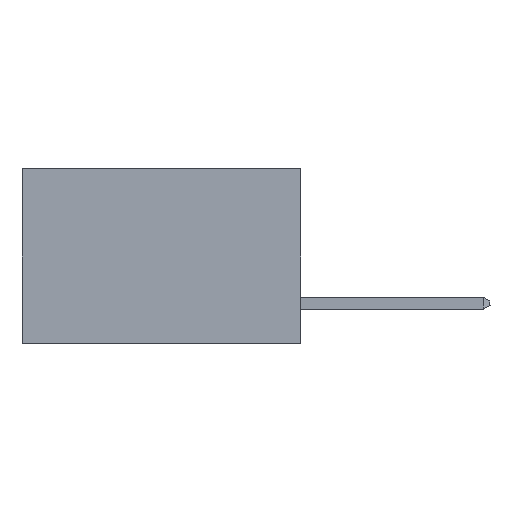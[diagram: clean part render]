
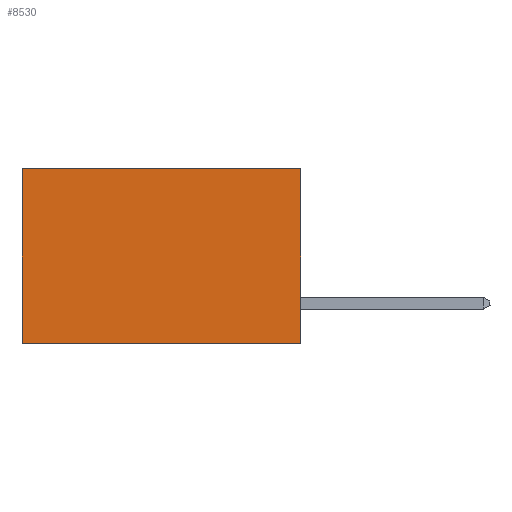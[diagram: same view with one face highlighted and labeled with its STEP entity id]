
A CAD part, left-side view. The second image highlights one B-rep face of the part: STEP entity #8530.
In plain terms, the highlighted planar face has unit normal (-1, 0, 0).
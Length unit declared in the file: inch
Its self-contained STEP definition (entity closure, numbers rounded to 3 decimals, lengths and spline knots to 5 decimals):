
#39 = ORIENTED_EDGE ( 'NONE', *, *, #13125, .T. ) ;
#360 = CARTESIAN_POINT ( 'NONE',  ( 0.277, 0.59, -0.37 ) ) ;
#2025 = CARTESIAN_POINT ( 'NONE',  ( 0.277, 0., -0.37 ) ) ;
#2088 = VECTOR ( 'NONE', #2269, 39.37008 ) ;
#2198 = CARTESIAN_POINT ( 'NONE',  ( 0.277, 0.59, 0. ) ) ;
#2269 = DIRECTION ( 'NONE',  ( 0., 0., -1. ) ) ;
#2933 = EDGE_CURVE ( 'NONE', #12472, #13410, #11295, .T. ) ;
#3009 = ORIENTED_EDGE ( 'NONE', *, *, #2933, .F. ) ;
#4418 = EDGE_CURVE ( 'NONE', #12472, #10656, #12048, .T. ) ;
#4995 = DIRECTION ( 'NONE',  ( 0., 0., -1. ) ) ;
#5043 = DIRECTION ( 'NONE',  ( 1., 0., 0. ) ) ;
#5099 = PLANE ( 'NONE',  #13318 ) ;
#5214 = CARTESIAN_POINT ( 'NONE',  ( 0.277, 0., -0.37 ) ) ;
#6611 = CARTESIAN_POINT ( 'NONE',  ( 0.277, 0., -0.37 ) ) ;
#7109 = CARTESIAN_POINT ( 'NONE',  ( 0.277, 0., -0.37 ) ) ;
#8530 = ADVANCED_FACE ( 'NONE', ( #11954 ), #5099, .F. ) ;
#9438 = CARTESIAN_POINT ( 'NONE',  ( 0.277, 0., 0. ) ) ;
#10656 = VERTEX_POINT ( 'NONE', #2198 ) ;
#11295 = LINE ( 'NONE', #2025, #11849 ) ;
#11760 = VECTOR ( 'NONE', #13800, 39.37008 ) ;
#11849 = VECTOR ( 'NONE', #16401, 39.37008 ) ;
#11954 = FACE_OUTER_BOUND ( 'NONE', #15161, .T. ) ;
#12048 = LINE ( 'NONE', #17544, #16717 ) ;
#12417 = ORIENTED_EDGE ( 'NONE', *, *, #13920, .F. ) ;
#12472 = VERTEX_POINT ( 'NONE', #9438 ) ;
#13125 = EDGE_CURVE ( 'NONE', #10656, #14734, #16491, .T. ) ;
#13318 = AXIS2_PLACEMENT_3D ( 'NONE', #5214, #5043, #4995 ) ;
#13410 = VERTEX_POINT ( 'NONE', #7109 ) ;
#13800 = DIRECTION ( 'NONE',  ( 0., 1., 0. ) ) ;
#13920 = EDGE_CURVE ( 'NONE', #13410, #14734, #21199, .T. ) ;
#14734 = VERTEX_POINT ( 'NONE', #22971 ) ;
#15161 = EDGE_LOOP ( 'NONE', ( #39, #12417, #3009, #23215 ) ) ;
#16401 = DIRECTION ( 'NONE',  ( 0., 0., -1. ) ) ;
#16491 = LINE ( 'NONE', #360, #2088 ) ;
#16717 = VECTOR ( 'NONE', #18313, 39.37008 ) ;
#17544 = CARTESIAN_POINT ( 'NONE',  ( 0.277, 0., 0. ) ) ;
#18313 = DIRECTION ( 'NONE',  ( 0., 1., 0. ) ) ;
#21199 = LINE ( 'NONE', #6611, #11760 ) ;
#22971 = CARTESIAN_POINT ( 'NONE',  ( 0.277, 0.59, -0.37 ) ) ;
#23215 = ORIENTED_EDGE ( 'NONE', *, *, #4418, .T. ) ;
